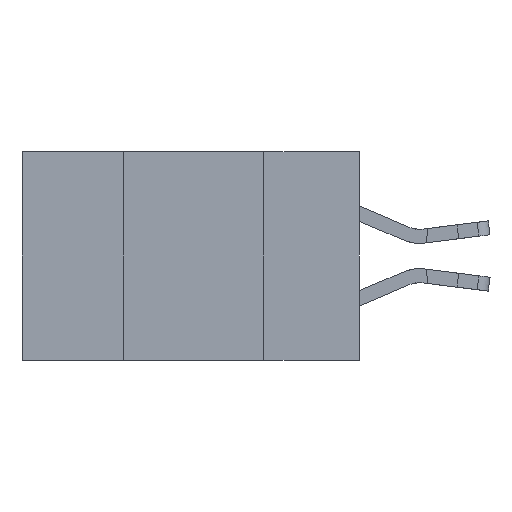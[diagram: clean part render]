
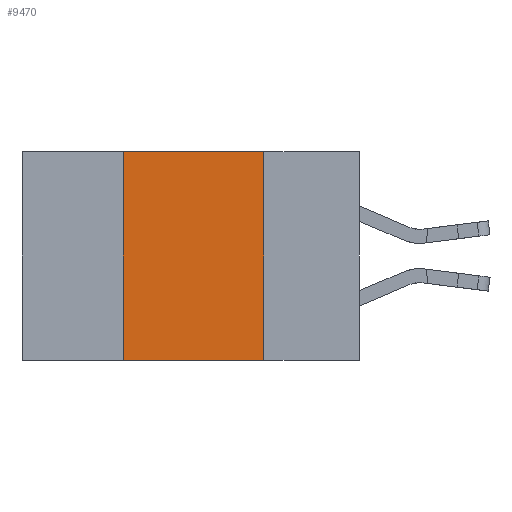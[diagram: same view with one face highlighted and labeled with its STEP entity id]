
A CAD part, left-side view. The second image highlights one B-rep face of the part: STEP entity #9470.
In plain terms, the highlighted planar face has unit normal (-1, 0, 0).
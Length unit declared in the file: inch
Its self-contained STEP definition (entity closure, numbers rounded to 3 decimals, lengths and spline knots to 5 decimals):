
#122 = LINE ( 'NONE', #12658, #6818 ) ;
#277 = LINE ( 'NONE', #2582, #14158 ) ;
#1011 = EDGE_LOOP ( 'NONE', ( #9488, #4022, #1721, #6987 ) ) ;
#1145 = DIRECTION ( 'NONE',  ( 0., 0., 1. ) ) ;
#1381 = FACE_OUTER_BOUND ( 'NONE', #1011, .T. ) ;
#1674 = DIRECTION ( 'NONE',  ( 0., -1., 0. ) ) ;
#1721 = ORIENTED_EDGE ( 'NONE', *, *, #5736, .F. ) ;
#2054 = EDGE_CURVE ( 'NONE', #9531, #15278, #277, .T. ) ;
#2582 = CARTESIAN_POINT ( 'NONE',  ( 0., 0.6, 0. ) ) ;
#2887 = AXIS2_PLACEMENT_3D ( 'NONE', #14093, #16763, #16824 ) ;
#4022 = ORIENTED_EDGE ( 'NONE', *, *, #2054, .F. ) ;
#4045 = CARTESIAN_POINT ( 'NONE',  ( 0., 0.17, -0.37 ) ) ;
#4719 = CARTESIAN_POINT ( 'NONE',  ( 0., 0.42, -0.37 ) ) ;
#4916 = PLANE ( 'NONE',  #2887 ) ;
#5736 = EDGE_CURVE ( 'NONE', #6487, #9531, #11141, .T. ) ;
#5778 = DIRECTION ( 'NONE',  ( 0., 0., -1. ) ) ;
#5832 = VECTOR ( 'NONE', #11533, 39.37008 ) ;
#6487 = VERTEX_POINT ( 'NONE', #4719 ) ;
#6818 = VECTOR ( 'NONE', #5778, 39.37008 ) ;
#6987 = ORIENTED_EDGE ( 'NONE', *, *, #7292, .T. ) ;
#7292 = EDGE_CURVE ( 'NONE', #6487, #16700, #11216, .T. ) ;
#7424 = CARTESIAN_POINT ( 'NONE',  ( 0., 0.42, 0. ) ) ;
#9095 = CARTESIAN_POINT ( 'NONE',  ( 0., 0.42, 0. ) ) ;
#9392 = EDGE_CURVE ( 'NONE', #15278, #16700, #122, .T. ) ;
#9470 = ADVANCED_FACE ( 'NONE', ( #1381 ), #4916, .F. ) ;
#9488 = ORIENTED_EDGE ( 'NONE', *, *, #9392, .F. ) ;
#9531 = VERTEX_POINT ( 'NONE', #7424 ) ;
#9796 = CARTESIAN_POINT ( 'NONE',  ( 0., 0.17, 0. ) ) ;
#10203 = CARTESIAN_POINT ( 'NONE',  ( 0., 0.6, -0.37 ) ) ;
#11141 = LINE ( 'NONE', #9095, #14256 ) ;
#11216 = LINE ( 'NONE', #10203, #5832 ) ;
#11533 = DIRECTION ( 'NONE',  ( 0., -1., 0. ) ) ;
#12658 = CARTESIAN_POINT ( 'NONE',  ( 0., 0.17, 0. ) ) ;
#14093 = CARTESIAN_POINT ( 'NONE',  ( 0., 0.6, 0. ) ) ;
#14158 = VECTOR ( 'NONE', #1674, 39.37008 ) ;
#14256 = VECTOR ( 'NONE', #1145, 39.37008 ) ;
#15278 = VERTEX_POINT ( 'NONE', #9796 ) ;
#16700 = VERTEX_POINT ( 'NONE', #4045 ) ;
#16763 = DIRECTION ( 'NONE',  ( 1., 0., 0. ) ) ;
#16824 = DIRECTION ( 'NONE',  ( 0., 0., -1. ) ) ;
